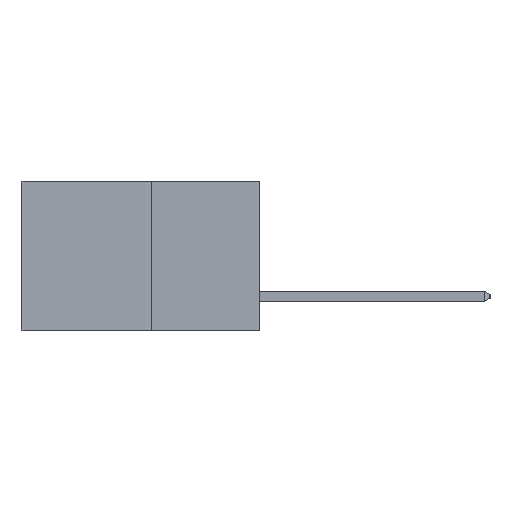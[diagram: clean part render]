
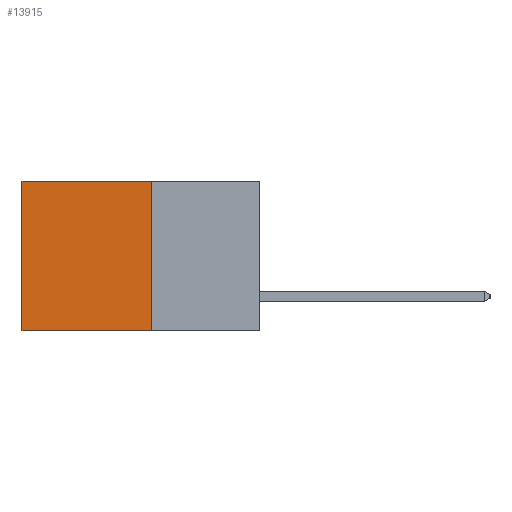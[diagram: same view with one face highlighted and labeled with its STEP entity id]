
A CAD part, left-side view. The second image highlights one B-rep face of the part: STEP entity #13915.
In plain terms, the highlighted planar face has unit normal (-1, 0, 0).
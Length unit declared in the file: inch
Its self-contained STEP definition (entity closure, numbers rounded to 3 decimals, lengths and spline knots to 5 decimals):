
#526 = LINE ( 'NONE', #6509, #13472 ) ;
#839 = DIRECTION ( 'NONE',  ( 0., 1., 0. ) ) ;
#1339 = CARTESIAN_POINT ( 'NONE',  ( 0.277, 0.59, 0. ) ) ;
#1828 = ORIENTED_EDGE ( 'NONE', *, *, #5099, .T. ) ;
#2627 = VERTEX_POINT ( 'NONE', #9595 ) ;
#2634 = EDGE_CURVE ( 'NONE', #2627, #14711, #13942, .T. ) ;
#2688 = ORIENTED_EDGE ( 'NONE', *, *, #2634, .T. ) ;
#3873 = DIRECTION ( 'NONE',  ( 0., 0., -1. ) ) ;
#3884 = VECTOR ( 'NONE', #839, 39.37008 ) ;
#5099 = EDGE_CURVE ( 'NONE', #14711, #6673, #526, .T. ) ;
#6509 = CARTESIAN_POINT ( 'NONE',  ( 0.277, 0.59, -0.37 ) ) ;
#6648 = DIRECTION ( 'NONE',  ( 0., 0., -1. ) ) ;
#6673 = VERTEX_POINT ( 'NONE', #16141 ) ;
#6738 = EDGE_LOOP ( 'NONE', ( #1828, #12144, #9270, #2688 ) ) ;
#7451 = FACE_OUTER_BOUND ( 'NONE', #6738, .T. ) ;
#7560 = EDGE_CURVE ( 'NONE', #2627, #11900, #7731, .T. ) ;
#7731 = LINE ( 'NONE', #11964, #13865 ) ;
#8112 = CARTESIAN_POINT ( 'NONE',  ( 0.277, 0.27, -0.37 ) ) ;
#9049 = PLANE ( 'NONE',  #10716 ) ;
#9225 = CARTESIAN_POINT ( 'NONE',  ( 0.277, 0.27, 0. ) ) ;
#9270 = ORIENTED_EDGE ( 'NONE', *, *, #7560, .F. ) ;
#9485 = DIRECTION ( 'NONE',  ( 0., 1., 0. ) ) ;
#9595 = CARTESIAN_POINT ( 'NONE',  ( 0.277, 0.27, 0. ) ) ;
#9598 = VECTOR ( 'NONE', #9485, 39.37008 ) ;
#10077 = EDGE_CURVE ( 'NONE', #11900, #6673, #16033, .T. ) ;
#10292 = CARTESIAN_POINT ( 'NONE',  ( 0.277, 0.27, -0.37 ) ) ;
#10660 = CARTESIAN_POINT ( 'NONE',  ( 0.277, 0.27, -0.37 ) ) ;
#10716 = AXIS2_PLACEMENT_3D ( 'NONE', #10292, #11497, #3873 ) ;
#10751 = DIRECTION ( 'NONE',  ( 0., 0., -1. ) ) ;
#11497 = DIRECTION ( 'NONE',  ( 1., 0., 0. ) ) ;
#11900 = VERTEX_POINT ( 'NONE', #8112 ) ;
#11964 = CARTESIAN_POINT ( 'NONE',  ( 0.277, 0.27, -0.37 ) ) ;
#12144 = ORIENTED_EDGE ( 'NONE', *, *, #10077, .F. ) ;
#13472 = VECTOR ( 'NONE', #6648, 39.37008 ) ;
#13865 = VECTOR ( 'NONE', #10751, 39.37008 ) ;
#13915 = ADVANCED_FACE ( 'NONE', ( #7451 ), #9049, .F. ) ;
#13942 = LINE ( 'NONE', #9225, #3884 ) ;
#14711 = VERTEX_POINT ( 'NONE', #1339 ) ;
#16033 = LINE ( 'NONE', #10660, #9598 ) ;
#16141 = CARTESIAN_POINT ( 'NONE',  ( 0.277, 0.59, -0.37 ) ) ;
